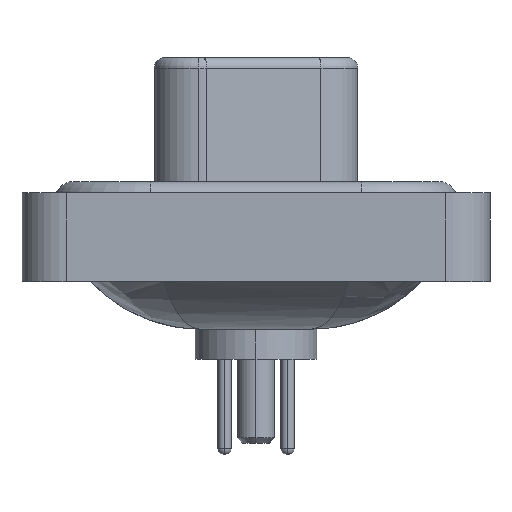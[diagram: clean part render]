
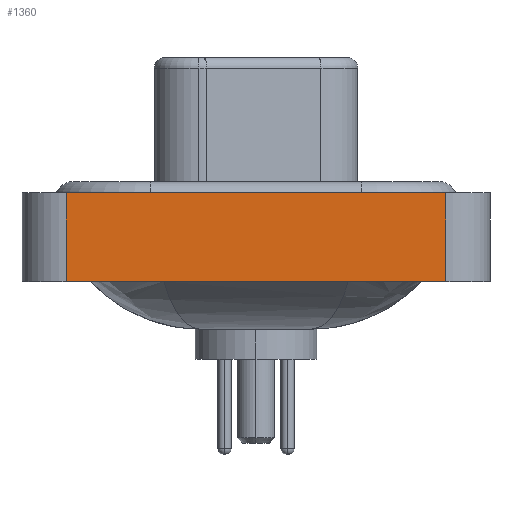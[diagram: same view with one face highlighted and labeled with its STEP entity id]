
A CAD part, left-side view. The second image highlights one B-rep face of the part: STEP entity #1360.
In plain terms, the highlighted planar face has unit normal (-1, 0, 0).
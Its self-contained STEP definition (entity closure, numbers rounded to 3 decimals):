
#1024 = ORIENTED_EDGE ( 'NONE', *, *, #19593, .T. ) ;
#1240 = CARTESIAN_POINT ( 'NONE',  ( -7.35, -8.55, 0.4 ) ) ;
#1360 = ADVANCED_FACE ( 'NONE', ( #2279 ), #2181, .T. ) ;
#2181 = PLANE ( 'NONE',  #2739 ) ;
#2255 = VECTOR ( 'NONE', #8781, 1000. ) ;
#2279 = FACE_OUTER_BOUND ( 'NONE', #10681, .T. ) ;
#2739 = AXIS2_PLACEMENT_3D ( 'NONE', #10021, #13302, #18082 ) ;
#3331 = ORIENTED_EDGE ( 'NONE', *, *, #12677, .T. ) ;
#3661 = CARTESIAN_POINT ( 'NONE',  ( -7.35, 8.55, -3.6 ) ) ;
#3776 = CARTESIAN_POINT ( 'NONE',  ( -7.35, -8.55, -3.6 ) ) ;
#3976 = VECTOR ( 'NONE', #19781, 1000. ) ;
#4852 = VERTEX_POINT ( 'NONE', #9419 ) ;
#4964 = VERTEX_POINT ( 'NONE', #3776 ) ;
#7157 = CARTESIAN_POINT ( 'NONE',  ( -7.35, 8.55, 0.4 ) ) ;
#8014 = CARTESIAN_POINT ( 'NONE',  ( -7.35, -8.55, 0.4 ) ) ;
#8781 = DIRECTION ( 'NONE',  ( 0., -1., 0. ) ) ;
#9419 = CARTESIAN_POINT ( 'NONE',  ( -7.35, 8.55, -3.6 ) ) ;
#9471 = EDGE_CURVE ( 'NONE', #4852, #18563, #14901, .T. ) ;
#9655 = CARTESIAN_POINT ( 'NONE',  ( -7.35, -8.55, -3.6 ) ) ;
#10021 = CARTESIAN_POINT ( 'NONE',  ( -7.35, -8.55, -3.6 ) ) ;
#10386 = EDGE_CURVE ( 'NONE', #18563, #14443, #19255, .T. ) ;
#10681 = EDGE_LOOP ( 'NONE', ( #1024, #15222, #10767, #3331 ) ) ;
#10767 = ORIENTED_EDGE ( 'NONE', *, *, #9471, .F. ) ;
#11790 = VECTOR ( 'NONE', #17442, 1000. ) ;
#12677 = EDGE_CURVE ( 'NONE', #4852, #4964, #16822, .T. ) ;
#12810 = VECTOR ( 'NONE', #14646, 1000. ) ;
#13302 = DIRECTION ( 'NONE',  ( -1., 0., 0. ) ) ;
#14443 = VERTEX_POINT ( 'NONE', #8014 ) ;
#14646 = DIRECTION ( 'NONE',  ( 0., 0., 1. ) ) ;
#14901 = LINE ( 'NONE', #3661, #3976 ) ;
#15222 = ORIENTED_EDGE ( 'NONE', *, *, #10386, .F. ) ;
#16822 = LINE ( 'NONE', #20230, #2255 ) ;
#17442 = DIRECTION ( 'NONE',  ( 0., -1., 0. ) ) ;
#18082 = DIRECTION ( 'NONE',  ( 0., 0., 1. ) ) ;
#18563 = VERTEX_POINT ( 'NONE', #7157 ) ;
#19255 = LINE ( 'NONE', #1240, #11790 ) ;
#19316 = LINE ( 'NONE', #9655, #12810 ) ;
#19593 = EDGE_CURVE ( 'NONE', #4964, #14443, #19316, .T. ) ;
#19781 = DIRECTION ( 'NONE',  ( 0., 0., 1. ) ) ;
#20230 = CARTESIAN_POINT ( 'NONE',  ( -7.35, -8.55, -3.6 ) ) ;
